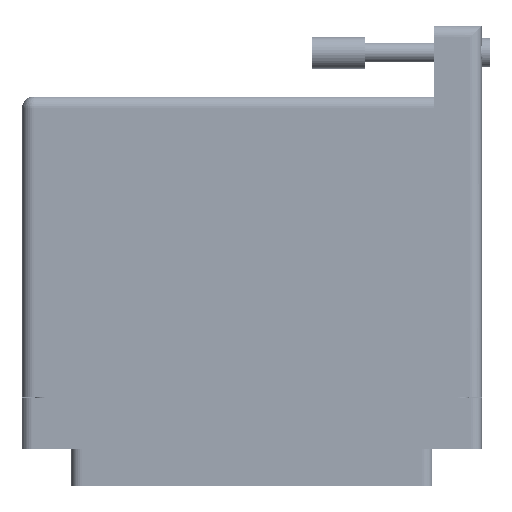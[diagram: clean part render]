
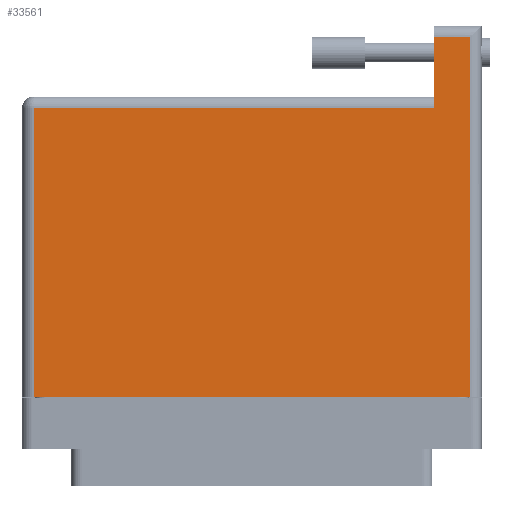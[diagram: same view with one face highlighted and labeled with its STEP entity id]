
A CAD part, front view. The second image highlights one B-rep face of the part: STEP entity #33561.
In plain terms, the highlighted face is planar.
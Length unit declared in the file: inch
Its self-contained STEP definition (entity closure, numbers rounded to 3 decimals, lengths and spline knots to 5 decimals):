
#593 = VECTOR ( 'NONE', #8966, 39.37008 ) ;
#2110 = VERTEX_POINT ( 'NONE', #43345 ) ;
#2271 = LINE ( 'NONE', #19641, #55647 ) ;
#3108 = DIRECTION ( 'NONE',  ( 1., 0., 0. ) ) ;
#3374 = EDGE_CURVE ( 'NONE', #10535, #19878, #40025, .T. ) ;
#4779 = VERTEX_POINT ( 'NONE', #42387 ) ;
#8380 = CARTESIAN_POINT ( 'NONE',  ( 1.289, 2.095, 0.617 ) ) ;
#8966 = DIRECTION ( 'NONE',  ( -1., 0., 0. ) ) ;
#8970 = EDGE_CURVE ( 'NONE', #22436, #4779, #13255, .T. ) ;
#10535 = VERTEX_POINT ( 'NONE', #24454 ) ;
#13255 = LINE ( 'NONE', #18937, #69126 ) ;
#14978 = LINE ( 'NONE', #30524, #30252 ) ;
#18937 = CARTESIAN_POINT ( 'NONE',  ( 1.079, 2.095, 0.617 ) ) ;
#19641 = CARTESIAN_POINT ( 'NONE',  ( -1.359, 1.605, 0.617 ) ) ;
#19878 = VERTEX_POINT ( 'NONE', #47205 ) ;
#22436 = VERTEX_POINT ( 'NONE', #67265 ) ;
#23577 = ORIENTED_EDGE ( 'NONE', *, *, #8970, .T. ) ;
#24077 = VECTOR ( 'NONE', #62959, 39.37008 ) ;
#24318 = DIRECTION ( 'NONE',  ( 0., -1., 0. ) ) ;
#24454 = CARTESIAN_POINT ( 'NONE',  ( -1.289, 1.605, 0.617 ) ) ;
#25213 = EDGE_CURVE ( 'NONE', #61782, #22436, #29386, .T. ) ;
#26980 = DIRECTION ( 'NONE',  ( -1., 0., 0. ) ) ;
#27807 = ORIENTED_EDGE ( 'NONE', *, *, #38695, .T. ) ;
#29386 = LINE ( 'NONE', #57260, #593 ) ;
#29514 = ORIENTED_EDGE ( 'NONE', *, *, #49657, .T. ) ;
#30252 = VECTOR ( 'NONE', #3108, 39.37008 ) ;
#30524 = CARTESIAN_POINT ( 'NONE',  ( -1.359, -0.1, 0.617 ) ) ;
#32365 = VECTOR ( 'NONE', #24318, 39.37008 ) ;
#33057 = ORIENTED_EDGE ( 'NONE', *, *, #25213, .T. ) ;
#33407 = ORIENTED_EDGE ( 'NONE', *, *, #36624, .T. ) ;
#33561 = ADVANCED_FACE ( 'NONE', ( #49299 ), #43211, .F. ) ;
#34327 = CARTESIAN_POINT ( 'NONE',  ( 1.289, 2.025, 0.617 ) ) ;
#36624 = EDGE_CURVE ( 'NONE', #4779, #10535, #2271, .T. ) ;
#38695 = EDGE_CURVE ( 'NONE', #2110, #61782, #64575, .T. ) ;
#40025 = LINE ( 'NONE', #45873, #32365 ) ;
#42387 = CARTESIAN_POINT ( 'NONE',  ( 1.079, 1.605, 0.617 ) ) ;
#43211 = PLANE ( 'NONE',  #63622 ) ;
#43345 = CARTESIAN_POINT ( 'NONE',  ( 1.289, -0.1, 0.617 ) ) ;
#45873 = CARTESIAN_POINT ( 'NONE',  ( -1.289, -0.1, 0.617 ) ) ;
#47205 = CARTESIAN_POINT ( 'NONE',  ( -1.289, -0.1, 0.617 ) ) ;
#48626 = DIRECTION ( 'NONE',  ( -1., 0., 0. ) ) ;
#49299 = FACE_OUTER_BOUND ( 'NONE', #65016, .T. ) ;
#49316 = DIRECTION ( 'NONE',  ( 0., 0., -1. ) ) ;
#49657 = EDGE_CURVE ( 'NONE', #19878, #2110, #14978, .T. ) ;
#55647 = VECTOR ( 'NONE', #26980, 39.37008 ) ;
#56576 = DIRECTION ( 'NONE',  ( 0., -1., 0. ) ) ;
#57260 = CARTESIAN_POINT ( 'NONE',  ( -1.359, 2.025, 0.617 ) ) ;
#59942 = ORIENTED_EDGE ( 'NONE', *, *, #3374, .T. ) ;
#61782 = VERTEX_POINT ( 'NONE', #34327 ) ;
#62959 = DIRECTION ( 'NONE',  ( 0., 1., 0. ) ) ;
#63622 = AXIS2_PLACEMENT_3D ( 'NONE', #64920, #49316, #48626 ) ;
#64575 = LINE ( 'NONE', #8380, #24077 ) ;
#64920 = CARTESIAN_POINT ( 'NONE',  ( -1.359, 1.675, 0.617 ) ) ;
#65016 = EDGE_LOOP ( 'NONE', ( #33407, #59942, #29514, #27807, #33057, #23577 ) ) ;
#67265 = CARTESIAN_POINT ( 'NONE',  ( 1.079, 2.025, 0.617 ) ) ;
#69126 = VECTOR ( 'NONE', #56576, 39.37008 ) ;
